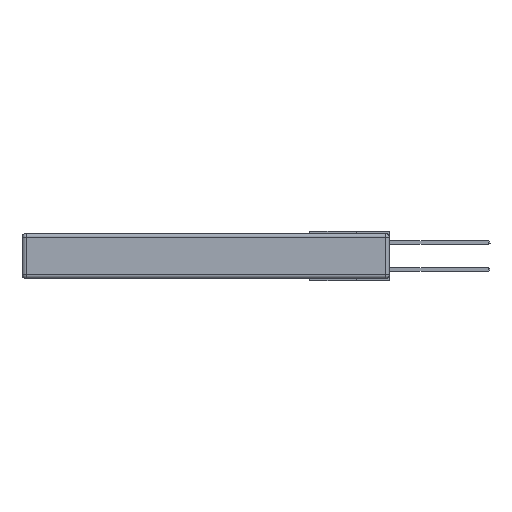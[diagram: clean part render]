
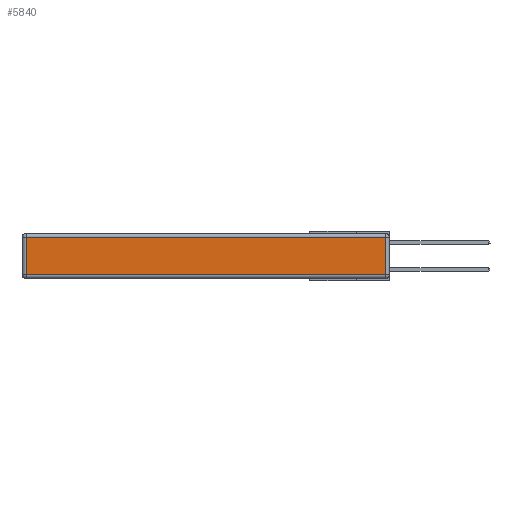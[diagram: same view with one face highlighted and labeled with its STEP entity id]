
A CAD part, left-side view. The second image highlights one B-rep face of the part: STEP entity #5840.
In plain terms, the highlighted planar face has unit normal (-1, 0, 0).
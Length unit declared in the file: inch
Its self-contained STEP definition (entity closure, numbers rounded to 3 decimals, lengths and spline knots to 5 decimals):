
#248 = PLANE ( 'NONE',  #29869 ) ;
#571 = CARTESIAN_POINT ( 'NONE',  ( 0., 0.03, -0.343 ) ) ;
#1100 = CARTESIAN_POINT ( 'NONE',  ( 0., 2.72, -0.313 ) ) ;
#1319 = VERTEX_POINT ( 'NONE', #23801 ) ;
#1775 = EDGE_CURVE ( 'NONE', #31353, #28886, #12452, .T. ) ;
#2247 = EDGE_CURVE ( 'NONE', #13698, #31353, #34226, .T. ) ;
#4934 = CARTESIAN_POINT ( 'NONE',  ( 0., 0., -0.313 ) ) ;
#5840 = ADVANCED_FACE ( 'NONE', ( #18806 ), #248, .T. ) ;
#7072 = LINE ( 'NONE', #4934, #15057 ) ;
#7413 = ORIENTED_EDGE ( 'NONE', *, *, #2247, .T. ) ;
#10740 = DIRECTION ( 'NONE',  ( 0., 0., -1. ) ) ;
#11847 = EDGE_CURVE ( 'NONE', #28886, #1319, #7072, .T. ) ;
#12452 = LINE ( 'NONE', #29363, #19171 ) ;
#13512 = CARTESIAN_POINT ( 'NONE',  ( 0., 2.75, -0.03 ) ) ;
#13698 = VERTEX_POINT ( 'NONE', #19242 ) ;
#14345 = CARTESIAN_POINT ( 'NONE',  ( 0., 2.72, -0.03 ) ) ;
#14876 = ORIENTED_EDGE ( 'NONE', *, *, #27734, .T. ) ;
#15057 = VECTOR ( 'NONE', #24314, 39.37008 ) ;
#16110 = EDGE_LOOP ( 'NONE', ( #32389, #14876, #7413, #20991 ) ) ;
#16168 = LINE ( 'NONE', #571, #20750 ) ;
#16216 = DIRECTION ( 'NONE',  ( -1., 0., 0. ) ) ;
#18806 = FACE_OUTER_BOUND ( 'NONE', #16110, .T. ) ;
#19171 = VECTOR ( 'NONE', #10740, 39.37008 ) ;
#19242 = CARTESIAN_POINT ( 'NONE',  ( 0., 0.03, -0.03 ) ) ;
#19330 = DIRECTION ( 'NONE',  ( 0., 0., 1. ) ) ;
#20750 = VECTOR ( 'NONE', #19330, 39.37008 ) ;
#20991 = ORIENTED_EDGE ( 'NONE', *, *, #1775, .T. ) ;
#21590 = DIRECTION ( 'NONE',  ( 0., 1., 0. ) ) ;
#21697 = CARTESIAN_POINT ( 'NONE',  ( 0., 0., -0.343 ) ) ;
#23801 = CARTESIAN_POINT ( 'NONE',  ( 0., 0.03, -0.313 ) ) ;
#24314 = DIRECTION ( 'NONE',  ( 0., -1., 0. ) ) ;
#27734 = EDGE_CURVE ( 'NONE', #1319, #13698, #16168, .T. ) ;
#28886 = VERTEX_POINT ( 'NONE', #1100 ) ;
#29363 = CARTESIAN_POINT ( 'NONE',  ( 0., 2.72, -0.343 ) ) ;
#29625 = VECTOR ( 'NONE', #21590, 39.37008 ) ;
#29869 = AXIS2_PLACEMENT_3D ( 'NONE', #21697, #16216, #32610 ) ;
#31353 = VERTEX_POINT ( 'NONE', #14345 ) ;
#32389 = ORIENTED_EDGE ( 'NONE', *, *, #11847, .T. ) ;
#32610 = DIRECTION ( 'NONE',  ( 0., 0., 1. ) ) ;
#34226 = LINE ( 'NONE', #13512, #29625 ) ;
